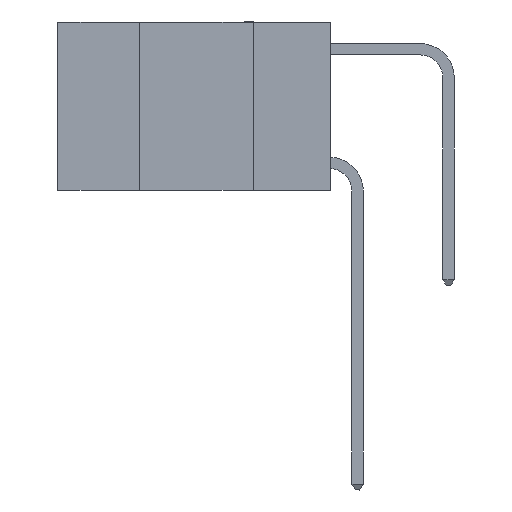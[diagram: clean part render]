
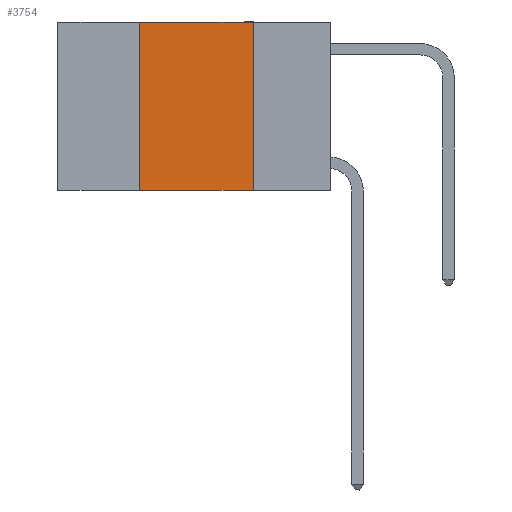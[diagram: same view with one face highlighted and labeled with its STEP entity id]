
A CAD part, left-side view. The second image highlights one B-rep face of the part: STEP entity #3754.
In plain terms, the highlighted planar face has unit normal (-1, 0, 0).
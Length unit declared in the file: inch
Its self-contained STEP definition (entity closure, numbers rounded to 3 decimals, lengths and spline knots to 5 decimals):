
#181 = VERTEX_POINT ( 'NONE', #20600 ) ;
#1283 = DIRECTION ( 'NONE',  ( 0., 0., -1. ) ) ;
#1349 = LINE ( 'NONE', #18322, #11040 ) ;
#2212 = LINE ( 'NONE', #5245, #12517 ) ;
#3333 = AXIS2_PLACEMENT_3D ( 'NONE', #23290, #14928, #19219 ) ;
#3754 = ADVANCED_FACE ( 'NONE', ( #13602 ), #8818, .F. ) ;
#4828 = CARTESIAN_POINT ( 'NONE',  ( 0., 0.42, 0. ) ) ;
#5207 = EDGE_CURVE ( 'NONE', #8728, #181, #1349, .T. ) ;
#5245 = CARTESIAN_POINT ( 'NONE',  ( 0., 0.17, 0. ) ) ;
#6598 = ORIENTED_EDGE ( 'NONE', *, *, #5207, .T. ) ;
#7088 = EDGE_CURVE ( 'NONE', #12130, #181, #2212, .T. ) ;
#7852 = DIRECTION ( 'NONE',  ( 0., -1., 0. ) ) ;
#7859 = CARTESIAN_POINT ( 'NONE',  ( 0., 0.42, 0. ) ) ;
#7944 = DIRECTION ( 'NONE',  ( 0., -1., 0. ) ) ;
#8728 = VERTEX_POINT ( 'NONE', #14407 ) ;
#8818 = PLANE ( 'NONE',  #3333 ) ;
#11040 = VECTOR ( 'NONE', #7852, 39.37008 ) ;
#11810 = VERTEX_POINT ( 'NONE', #7859 ) ;
#12130 = VERTEX_POINT ( 'NONE', #15031 ) ;
#12517 = VECTOR ( 'NONE', #1283, 39.37008 ) ;
#12687 = VECTOR ( 'NONE', #7944, 39.37008 ) ;
#13602 = FACE_OUTER_BOUND ( 'NONE', #21904, .T. ) ;
#14270 = ORIENTED_EDGE ( 'NONE', *, *, #15011, .F. ) ;
#14407 = CARTESIAN_POINT ( 'NONE',  ( 0., 0.42, -0.37 ) ) ;
#14927 = VECTOR ( 'NONE', #19107, 39.37008 ) ;
#14928 = DIRECTION ( 'NONE',  ( 1., 0., 0. ) ) ;
#15011 = EDGE_CURVE ( 'NONE', #8728, #11810, #15266, .T. ) ;
#15031 = CARTESIAN_POINT ( 'NONE',  ( 0., 0.17, 0. ) ) ;
#15266 = LINE ( 'NONE', #4828, #14927 ) ;
#18161 = CARTESIAN_POINT ( 'NONE',  ( 0., 0.6, 0. ) ) ;
#18219 = LINE ( 'NONE', #18161, #12687 ) ;
#18322 = CARTESIAN_POINT ( 'NONE',  ( 0., 0.6, -0.37 ) ) ;
#19107 = DIRECTION ( 'NONE',  ( 0., 0., 1. ) ) ;
#19219 = DIRECTION ( 'NONE',  ( 0., 0., -1. ) ) ;
#19860 = ORIENTED_EDGE ( 'NONE', *, *, #22196, .F. ) ;
#20600 = CARTESIAN_POINT ( 'NONE',  ( 0., 0.17, -0.37 ) ) ;
#21904 = EDGE_LOOP ( 'NONE', ( #26620, #19860, #14270, #6598 ) ) ;
#22196 = EDGE_CURVE ( 'NONE', #11810, #12130, #18219, .T. ) ;
#23290 = CARTESIAN_POINT ( 'NONE',  ( 0., 0.6, 0. ) ) ;
#26620 = ORIENTED_EDGE ( 'NONE', *, *, #7088, .F. ) ;
